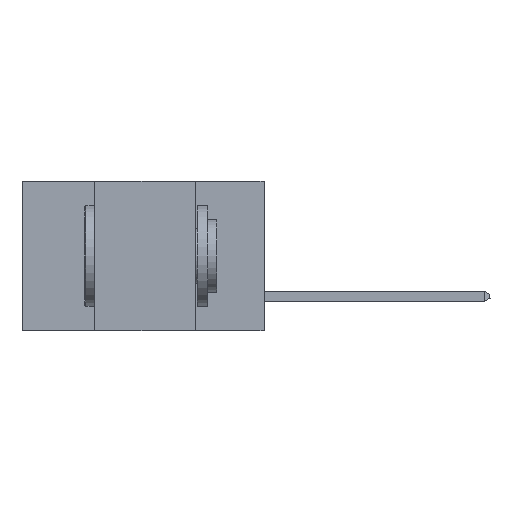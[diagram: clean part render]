
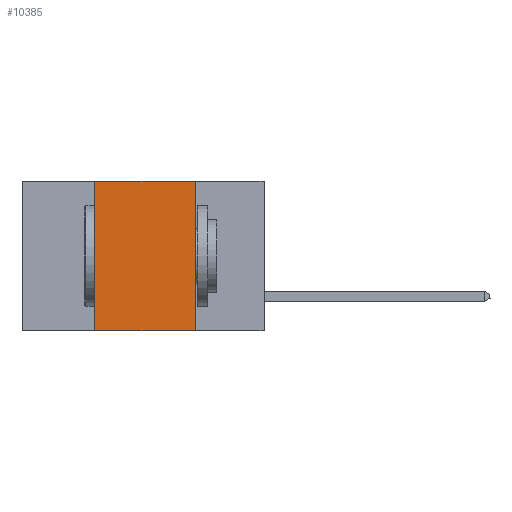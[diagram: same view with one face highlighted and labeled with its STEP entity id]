
A CAD part, left-side view. The second image highlights one B-rep face of the part: STEP entity #10385.
In plain terms, the highlighted planar face has unit normal (-1, 0, 0).
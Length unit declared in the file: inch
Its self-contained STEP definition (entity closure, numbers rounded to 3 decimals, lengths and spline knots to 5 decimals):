
#734 = AXIS2_PLACEMENT_3D ( 'NONE', #3104, #5858, #2237 ) ;
#1055 = VERTEX_POINT ( 'NONE', #11499 ) ;
#1111 = EDGE_CURVE ( 'NONE', #1055, #6571, #3146, .T. ) ;
#1551 = VECTOR ( 'NONE', #7234, 39.37008 ) ;
#1623 = EDGE_CURVE ( 'NONE', #6571, #6312, #4181, .T. ) ;
#2237 = DIRECTION ( 'NONE',  ( 0., 0., -1. ) ) ;
#2261 = VECTOR ( 'NONE', #6793, 39.37008 ) ;
#2294 = CARTESIAN_POINT ( 'NONE',  ( 0., 0.6, -0.37 ) ) ;
#3104 = CARTESIAN_POINT ( 'NONE',  ( 0., 0.6, 0. ) ) ;
#3146 = LINE ( 'NONE', #4882, #2261 ) ;
#3901 = DIRECTION ( 'NONE',  ( 0., 0., 1. ) ) ;
#4181 = LINE ( 'NONE', #7626, #7302 ) ;
#4217 = CARTESIAN_POINT ( 'NONE',  ( 0., 0.17, 0. ) ) ;
#4398 = EDGE_LOOP ( 'NONE', ( #7439, #4813, #7005, #7704 ) ) ;
#4697 = FACE_OUTER_BOUND ( 'NONE', #4398, .T. ) ;
#4813 = ORIENTED_EDGE ( 'NONE', *, *, #1111, .F. ) ;
#4882 = CARTESIAN_POINT ( 'NONE',  ( 0., 0.6, 0. ) ) ;
#5141 = LINE ( 'NONE', #2294, #1551 ) ;
#5649 = VECTOR ( 'NONE', #3901, 39.37008 ) ;
#5858 = DIRECTION ( 'NONE',  ( 1., 0., 0. ) ) ;
#6312 = VERTEX_POINT ( 'NONE', #7763 ) ;
#6526 = CARTESIAN_POINT ( 'NONE',  ( 0., 0.42, 0. ) ) ;
#6537 = CARTESIAN_POINT ( 'NONE',  ( 0., 0.42, -0.37 ) ) ;
#6571 = VERTEX_POINT ( 'NONE', #4217 ) ;
#6793 = DIRECTION ( 'NONE',  ( 0., -1., 0. ) ) ;
#7005 = ORIENTED_EDGE ( 'NONE', *, *, #7342, .F. ) ;
#7234 = DIRECTION ( 'NONE',  ( 0., -1., 0. ) ) ;
#7302 = VECTOR ( 'NONE', #7587, 39.37008 ) ;
#7342 = EDGE_CURVE ( 'NONE', #12145, #1055, #11159, .T. ) ;
#7439 = ORIENTED_EDGE ( 'NONE', *, *, #1623, .F. ) ;
#7587 = DIRECTION ( 'NONE',  ( 0., 0., -1. ) ) ;
#7626 = CARTESIAN_POINT ( 'NONE',  ( 0., 0.17, 0. ) ) ;
#7704 = ORIENTED_EDGE ( 'NONE', *, *, #11266, .T. ) ;
#7763 = CARTESIAN_POINT ( 'NONE',  ( 0., 0.17, -0.37 ) ) ;
#7911 = PLANE ( 'NONE',  #734 ) ;
#10385 = ADVANCED_FACE ( 'NONE', ( #4697 ), #7911, .F. ) ;
#11159 = LINE ( 'NONE', #6526, #5649 ) ;
#11266 = EDGE_CURVE ( 'NONE', #12145, #6312, #5141, .T. ) ;
#11499 = CARTESIAN_POINT ( 'NONE',  ( 0., 0.42, 0. ) ) ;
#12145 = VERTEX_POINT ( 'NONE', #6537 ) ;
